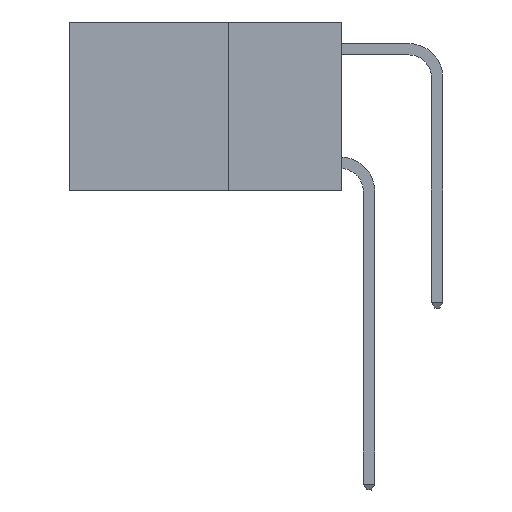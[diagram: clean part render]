
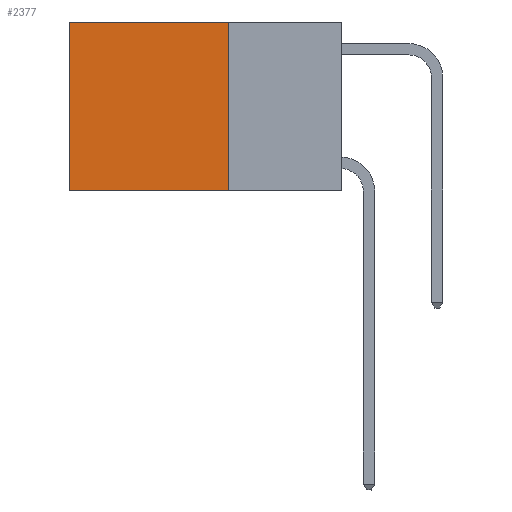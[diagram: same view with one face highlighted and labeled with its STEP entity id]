
A CAD part, left-side view. The second image highlights one B-rep face of the part: STEP entity #2377.
In plain terms, the highlighted planar face has unit normal (-1, 0, 0).
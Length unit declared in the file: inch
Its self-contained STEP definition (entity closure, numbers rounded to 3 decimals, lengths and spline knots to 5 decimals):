
#61 = VECTOR ( 'NONE', #4500, 39.37008 ) ;
#100 = LINE ( 'NONE', #8947, #9529 ) ;
#1999 = EDGE_LOOP ( 'NONE', ( #18343, #18555, #13325, #20028 ) ) ;
#2188 = VERTEX_POINT ( 'NONE', #6002 ) ;
#2377 = ADVANCED_FACE ( 'NONE', ( #21153 ), #11503, .F. ) ;
#3068 = CARTESIAN_POINT ( 'NONE',  ( 0.2625, 0.25, -0.37 ) ) ;
#3710 = VECTOR ( 'NONE', #16895, 39.37008 ) ;
#4500 = DIRECTION ( 'NONE',  ( 0., 1., 0. ) ) ;
#5280 = VERTEX_POINT ( 'NONE', #14303 ) ;
#5290 = CARTESIAN_POINT ( 'NONE',  ( 0.2625, 0.6, 0. ) ) ;
#6002 = CARTESIAN_POINT ( 'NONE',  ( 0.2625, 0.6, -0.37 ) ) ;
#6506 = CARTESIAN_POINT ( 'NONE',  ( 0.2625, 0.25, 0. ) ) ;
#7126 = LINE ( 'NONE', #5290, #3710 ) ;
#7445 = AXIS2_PLACEMENT_3D ( 'NONE', #6506, #19745, #9890 ) ;
#8631 = VERTEX_POINT ( 'NONE', #14348 ) ;
#8947 = CARTESIAN_POINT ( 'NONE',  ( 0.2625, 0.25, -0.37 ) ) ;
#9529 = VECTOR ( 'NONE', #20464, 39.37008 ) ;
#9890 = DIRECTION ( 'NONE',  ( 0., 0., -1. ) ) ;
#11503 = PLANE ( 'NONE',  #7445 ) ;
#12901 = LINE ( 'NONE', #16124, #61 ) ;
#12953 = EDGE_CURVE ( 'NONE', #5280, #17049, #13844, .T. ) ;
#13325 = ORIENTED_EDGE ( 'NONE', *, *, #12953, .F. ) ;
#13844 = LINE ( 'NONE', #18193, #17663 ) ;
#14111 = EDGE_CURVE ( 'NONE', #17049, #2188, #100, .T. ) ;
#14303 = CARTESIAN_POINT ( 'NONE',  ( 0.2625, 0.25, 0. ) ) ;
#14348 = CARTESIAN_POINT ( 'NONE',  ( 0.2625, 0.6, 0. ) ) ;
#15567 = EDGE_CURVE ( 'NONE', #5280, #8631, #12901, .T. ) ;
#15858 = EDGE_CURVE ( 'NONE', #8631, #2188, #7126, .T. ) ;
#16124 = CARTESIAN_POINT ( 'NONE',  ( 0.2625, 0.25, 0. ) ) ;
#16551 = DIRECTION ( 'NONE',  ( 0., 0., -1. ) ) ;
#16895 = DIRECTION ( 'NONE',  ( 0., 0., -1. ) ) ;
#17049 = VERTEX_POINT ( 'NONE', #3068 ) ;
#17663 = VECTOR ( 'NONE', #16551, 39.37008 ) ;
#18193 = CARTESIAN_POINT ( 'NONE',  ( 0.2625, 0.25, 0. ) ) ;
#18343 = ORIENTED_EDGE ( 'NONE', *, *, #15858, .T. ) ;
#18555 = ORIENTED_EDGE ( 'NONE', *, *, #14111, .F. ) ;
#19745 = DIRECTION ( 'NONE',  ( 1., 0., 0. ) ) ;
#20028 = ORIENTED_EDGE ( 'NONE', *, *, #15567, .T. ) ;
#20464 = DIRECTION ( 'NONE',  ( 0., 1., 0. ) ) ;
#21153 = FACE_OUTER_BOUND ( 'NONE', #1999, .T. ) ;
